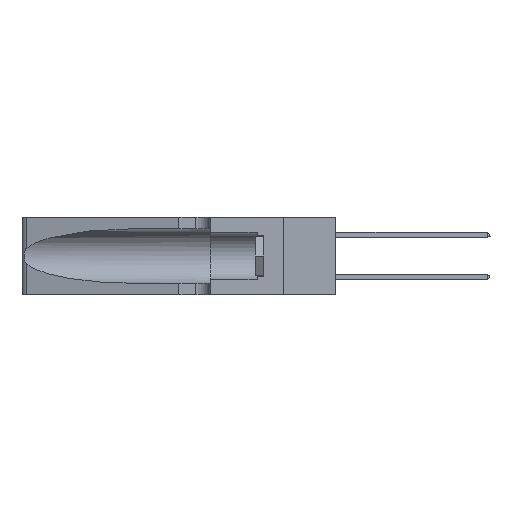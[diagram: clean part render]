
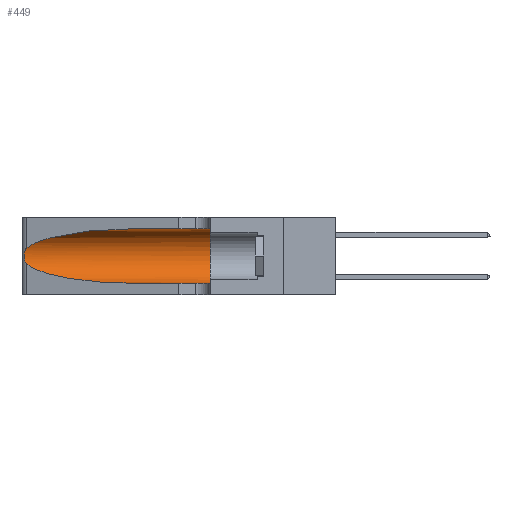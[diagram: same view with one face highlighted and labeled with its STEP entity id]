
A CAD part, left-side view. The second image highlights one B-rep face of the part: STEP entity #449.
In plain terms, the highlighted cylindrical face has radius 3.308 mm (diameter 6.617 mm), a partial arc.
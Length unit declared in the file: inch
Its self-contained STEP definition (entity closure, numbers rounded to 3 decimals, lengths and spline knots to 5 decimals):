
#23 = VERTEX_POINT ( 'NONE', #1975 ) ;
#449 = ADVANCED_FACE ( 'NONE', ( #8897 ), #11113, .F. ) ;
#692 = DIRECTION ( 'NONE',  ( 0., -1., 0. ) ) ;
#1057 = CARTESIAN_POINT ( 'NONE',  ( 0.18966, 0.96281, 0.31525 ) ) ;
#1174 = VECTOR ( 'NONE', #3501, 39.37008 ) ;
#1935 = CARTESIAN_POINT ( 'NONE',  ( 0.25487, 1.22718, 0.14631 ) ) ;
#1975 = CARTESIAN_POINT ( 'NONE',  ( 0.25487, 1.22718, 0.14631 ) ) ;
#2283 = VERTEX_POINT ( 'NONE', #6189 ) ;
#2691 = VERTEX_POINT ( 'NONE', #3914 ) ;
#3050 = CARTESIAN_POINT ( 'NONE',  ( 0.25555, 1.22994, 0.2215 ) ) ;
#3086 = VECTOR ( 'NONE', #692, 39.37008 ) ;
#3138 = CARTESIAN_POINT ( 'NONE',  ( 0.26075, 1.23896, 0.178 ) ) ;
#3501 = DIRECTION ( 'NONE',  ( 0., -1., 0. ) ) ;
#3914 = CARTESIAN_POINT ( 'NONE',  ( 0.25487, 1.22718, 0.22369 ) ) ;
#4049 = AXIS2_PLACEMENT_3D ( 'NONE', #20742, #25730, #23939 ) ;
#4318 = CARTESIAN_POINT ( 'NONE',  ( 0.18966, 0.96281, 0.05475 ) ) ;
#4848 = ORIENTED_EDGE ( 'NONE', *, *, #16834, .F. ) ;
#5615 =( BOUNDED_CURVE ( )  B_SPLINE_CURVE ( 3, ( #23500, #1057, #17204, #7101 ),
 .UNSPECIFIED., .F., .F. ) 
 B_SPLINE_CURVE_WITH_KNOTS ( ( 4, 4 ),
 ( 1.5708, 2.84003 ),
 .UNSPECIFIED. ) 
 CURVE ( )  GEOMETRIC_REPRESENTATION_ITEM ( )  RATIONAL_B_SPLINE_CURVE ( ( 1., 0.87, 0.87, 1. ) ) 
 REPRESENTATION_ITEM ( '' )  );
#5695 = EDGE_LOOP ( 'NONE', ( #7063, #17362, #9880, #20500, #21502, #4848 ) ) ;
#5696 = CARTESIAN_POINT ( 'NONE',  ( 0.1305, 0.35, 0.05475 ) ) ;
#6189 = CARTESIAN_POINT ( 'NONE',  ( 0.1305, 0.35, 0.31525 ) ) ;
#6729 =( BOUNDED_CURVE ( )  B_SPLINE_CURVE ( 3, ( #1935, #24729, #4318, #15654 ),
 .UNSPECIFIED., .F., .F. ) 
 B_SPLINE_CURVE_WITH_KNOTS ( ( 4, 4 ),
 ( 3.44316, 4.71239 ),
 .UNSPECIFIED. ) 
 CURVE ( )  GEOMETRIC_REPRESENTATION_ITEM ( )  RATIONAL_B_SPLINE_CURVE ( ( 1., 0.87, 0.87, 1. ) ) 
 REPRESENTATION_ITEM ( '' )  );
#7063 = ORIENTED_EDGE ( 'NONE', *, *, #7767, .T. ) ;
#7099 = AXIS2_PLACEMENT_3D ( 'NONE', #20479, #16347, #14509 ) ;
#7101 = CARTESIAN_POINT ( 'NONE',  ( 0.25487, 1.22718, 0.22369 ) ) ;
#7104 = CARTESIAN_POINT ( 'NONE',  ( 0.25787, 1.23484, 0.2124 ) ) ;
#7200 = CARTESIAN_POINT ( 'NONE',  ( 0.25789, 1.23486, 0.15765 ) ) ;
#7767 = EDGE_CURVE ( 'NONE', #13603, #2691, #5615, .T. ) ;
#7888 = LINE ( 'NONE', #15688, #1174 ) ;
#8210 = VERTEX_POINT ( 'NONE', #5696 ) ;
#8491 = EDGE_CURVE ( 'NONE', #23, #10759, #6729, .T. ) ;
#8897 = FACE_OUTER_BOUND ( 'NONE', #5695, .T. ) ;
#9880 = ORIENTED_EDGE ( 'NONE', *, *, #8491, .T. ) ;
#10540 = CIRCLE ( 'NONE', #7099, 0.13025 ) ;
#10739 = CARTESIAN_POINT ( 'NONE',  ( 0.1305, 0.72297, 0.31525 ) ) ;
#10759 = VERTEX_POINT ( 'NONE', #23038 ) ;
#11105 = CARTESIAN_POINT ( 'NONE',  ( 0.25487, 1.22718, 0.22369 ) ) ;
#11113 = CYLINDRICAL_SURFACE ( 'NONE', #4049, 0.13025 ) ;
#11288 = CARTESIAN_POINT ( 'NONE',  ( 0.25555, 1.22993, 0.14849 ) ) ;
#11652 = LINE ( 'NONE', #12692, #3086 ) ;
#12692 = CARTESIAN_POINT ( 'NONE',  ( 0.1305, 1.61858, 0.31525 ) ) ;
#13229 = CARTESIAN_POINT ( 'NONE',  ( 0.26018, 1.23835, 0.19895 ) ) ;
#13314 = CARTESIAN_POINT ( 'NONE',  ( 0.25487, 1.22718, 0.14631 ) ) ;
#13603 = VERTEX_POINT ( 'NONE', #10739 ) ;
#14509 = DIRECTION ( 'NONE',  ( 0., 0., 1. ) ) ;
#15303 = CARTESIAN_POINT ( 'NONE',  ( 0.26075, 1.23896, 0.19203 ) ) ;
#15654 = CARTESIAN_POINT ( 'NONE',  ( 0.1305, 0.72297, 0.05475 ) ) ;
#15688 = CARTESIAN_POINT ( 'NONE',  ( 0.1305, 1.61858, 0.05475 ) ) ;
#16347 = DIRECTION ( 'NONE',  ( 0., 1., 0. ) ) ;
#16480 = EDGE_CURVE ( 'NONE', #10759, #8210, #7888, .T. ) ;
#16834 = EDGE_CURVE ( 'NONE', #13603, #2283, #11652, .T. ) ;
#17044 = B_SPLINE_CURVE_WITH_KNOTS ( 'NONE', 3,
 ( #11105, #3050, #19346, #7104, #23504, #13229, #15303, #3138, #17394, #19437, #7200, #23600, #11288, #13314 ),
 .UNSPECIFIED., .F., .F.,
 ( 4, 2, 2, 2, 2, 2, 4 ),
 ( 0., 0.00027, 0.00053, 0.00107, 0.0016, 0.00187, 0.00214 ),
 .UNSPECIFIED. ) ;
#17204 = CARTESIAN_POINT ( 'NONE',  ( 0.2373, 1.15595, 0.28018 ) ) ;
#17362 = ORIENTED_EDGE ( 'NONE', *, *, #24990, .T. ) ;
#17394 = CARTESIAN_POINT ( 'NONE',  ( 0.26017, 1.23833, 0.17102 ) ) ;
#19346 = CARTESIAN_POINT ( 'NONE',  ( 0.25639, 1.23184, 0.21858 ) ) ;
#19437 = CARTESIAN_POINT ( 'NONE',  ( 0.25856, 1.23593, 0.16098 ) ) ;
#20479 = CARTESIAN_POINT ( 'NONE',  ( 0.1305, 0.35, 0.185 ) ) ;
#20500 = ORIENTED_EDGE ( 'NONE', *, *, #16480, .T. ) ;
#20742 = CARTESIAN_POINT ( 'NONE',  ( 0.1305, 1.61858, 0.185 ) ) ;
#21502 = ORIENTED_EDGE ( 'NONE', *, *, #22523, .F. ) ;
#22523 = EDGE_CURVE ( 'NONE', #2283, #8210, #10540, .T. ) ;
#23038 = CARTESIAN_POINT ( 'NONE',  ( 0.1305, 0.72297, 0.05475 ) ) ;
#23500 = CARTESIAN_POINT ( 'NONE',  ( 0.1305, 0.72297, 0.31525 ) ) ;
#23504 = CARTESIAN_POINT ( 'NONE',  ( 0.25854, 1.2359, 0.20912 ) ) ;
#23600 = CARTESIAN_POINT ( 'NONE',  ( 0.25639, 1.23186, 0.15144 ) ) ;
#23939 = DIRECTION ( 'NONE',  ( 0., 0., -1. ) ) ;
#24729 = CARTESIAN_POINT ( 'NONE',  ( 0.2373, 1.15595, 0.08982 ) ) ;
#24990 = EDGE_CURVE ( 'NONE', #2691, #23, #17044, .T. ) ;
#25730 = DIRECTION ( 'NONE',  ( 0., -1., 0. ) ) ;
